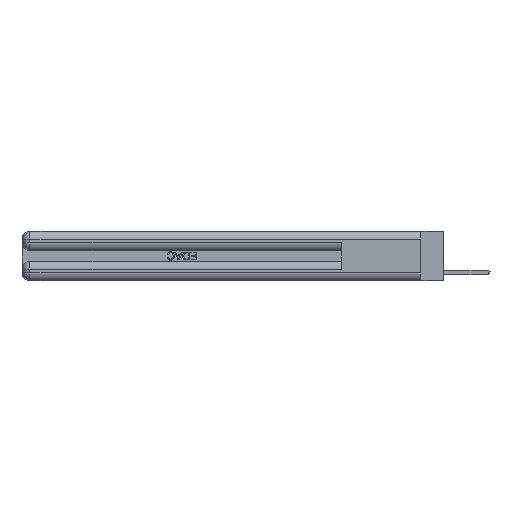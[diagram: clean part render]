
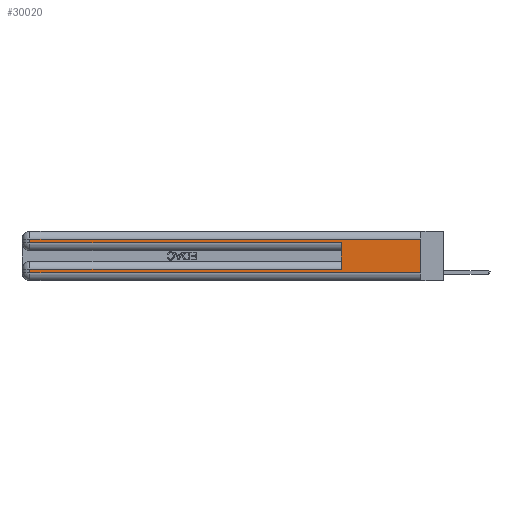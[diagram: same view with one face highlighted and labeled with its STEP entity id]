
A CAD part, left-side view. The second image highlights one B-rep face of the part: STEP entity #30020.
In plain terms, the highlighted planar face has unit normal (-1, 0, 0).
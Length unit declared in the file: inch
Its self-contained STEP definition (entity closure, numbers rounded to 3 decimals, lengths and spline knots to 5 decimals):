
#575 = ORIENTED_EDGE ( 'NONE', *, *, #23349, .F. ) ;
#660 = DIRECTION ( 'NONE',  ( 0., 0., 1. ) ) ;
#1958 = ORIENTED_EDGE ( 'NONE', *, *, #13473, .T. ) ;
#2178 = EDGE_CURVE ( 'NONE', #5059, #28008, #10118, .T. ) ;
#2394 = VECTOR ( 'NONE', #660, 39.37008 ) ;
#2495 = LINE ( 'NONE', #28768, #8715 ) ;
#2496 = FACE_OUTER_BOUND ( 'NONE', #28478, .T. ) ;
#2797 = CARTESIAN_POINT ( 'NONE',  ( 0., 0.6, 0.145 ) ) ;
#2930 = DIRECTION ( 'NONE',  ( 0., -1., 0. ) ) ;
#3927 = DIRECTION ( 'NONE',  ( 0., 0., -1. ) ) ;
#5059 = VERTEX_POINT ( 'NONE', #8813 ) ;
#5976 = CARTESIAN_POINT ( 'NONE',  ( 0., 2.94, 0.37 ) ) ;
#6125 = DIRECTION ( 'NONE',  ( 0., 0., -1. ) ) ;
#7671 = EDGE_CURVE ( 'NONE', #9877, #20302, #30040, .T. ) ;
#7753 = CARTESIAN_POINT ( 'NONE',  ( 0., 2.94, 0.285 ) ) ;
#7903 = CARTESIAN_POINT ( 'NONE',  ( 0., 0., 0.085 ) ) ;
#8715 = VECTOR ( 'NONE', #10646, 39.37008 ) ;
#8813 = CARTESIAN_POINT ( 'NONE',  ( 0., 0.6, 0.085 ) ) ;
#9092 = DIRECTION ( 'NONE',  ( 0., -1., 0. ) ) ;
#9561 = DIRECTION ( 'NONE',  ( 0., 1., 0. ) ) ;
#9877 = VERTEX_POINT ( 'NONE', #28193 ) ;
#10118 = LINE ( 'NONE', #7903, #12491 ) ;
#10181 = DIRECTION ( 'NONE',  ( 1., 0., 0. ) ) ;
#10646 = DIRECTION ( 'NONE',  ( 0., 0., -1. ) ) ;
#11634 = ORIENTED_EDGE ( 'NONE', *, *, #19219, .T. ) ;
#12491 = VECTOR ( 'NONE', #15438, 39.37008 ) ;
#12512 = CARTESIAN_POINT ( 'NONE',  ( 0., 0., 0.37 ) ) ;
#12623 = ORIENTED_EDGE ( 'NONE', *, *, #7671, .F. ) ;
#13065 = ORIENTED_EDGE ( 'NONE', *, *, #20601, .T. ) ;
#13370 = VECTOR ( 'NONE', #9092, 39.37008 ) ;
#13473 = EDGE_CURVE ( 'NONE', #28131, #22437, #15703, .T. ) ;
#15438 = DIRECTION ( 'NONE',  ( 0., 1., 0. ) ) ;
#15703 = LINE ( 'NONE', #5976, #20096 ) ;
#16310 = VECTOR ( 'NONE', #9561, 39.37008 ) ;
#16314 = CARTESIAN_POINT ( 'NONE',  ( 0., 0., 0.285 ) ) ;
#17798 = VERTEX_POINT ( 'NONE', #25293 ) ;
#18043 = EDGE_CURVE ( 'NONE', #17798, #20302, #19240, .T. ) ;
#18176 = EDGE_CURVE ( 'NONE', #28008, #17798, #2495, .T. ) ;
#18614 = AXIS2_PLACEMENT_3D ( 'NONE', #12512, #10181, #26714 ) ;
#19219 = EDGE_CURVE ( 'NONE', #9877, #28131, #23289, .T. ) ;
#19240 = LINE ( 'NONE', #26866, #30184 ) ;
#19350 = ORIENTED_EDGE ( 'NONE', *, *, #2178, .T. ) ;
#20096 = VECTOR ( 'NONE', #6125, 39.37008 ) ;
#20302 = VERTEX_POINT ( 'NONE', #21498 ) ;
#20580 = ORIENTED_EDGE ( 'NONE', *, *, #18176, .T. ) ;
#20601 = EDGE_CURVE ( 'NONE', #22437, #27794, #21268, .T. ) ;
#20970 = CARTESIAN_POINT ( 'NONE',  ( 0., 0., 0.37 ) ) ;
#21268 = LINE ( 'NONE', #16314, #13370 ) ;
#21498 = CARTESIAN_POINT ( 'NONE',  ( 0., 0., 0.06 ) ) ;
#22437 = VERTEX_POINT ( 'NONE', #7753 ) ;
#23289 = LINE ( 'NONE', #23753, #16310 ) ;
#23349 = EDGE_CURVE ( 'NONE', #5059, #27794, #24363, .T. ) ;
#23753 = CARTESIAN_POINT ( 'NONE',  ( 0., 0., 0.31 ) ) ;
#23778 = CARTESIAN_POINT ( 'NONE',  ( 0., 2.94, 0.31 ) ) ;
#23960 = CARTESIAN_POINT ( 'NONE',  ( 0., 0.6, 0.285 ) ) ;
#24363 = LINE ( 'NONE', #2797, #2394 ) ;
#25293 = CARTESIAN_POINT ( 'NONE',  ( 0., 2.94, 0.06 ) ) ;
#26714 = DIRECTION ( 'NONE',  ( 0., 0., -1. ) ) ;
#26866 = CARTESIAN_POINT ( 'NONE',  ( 0., 0., 0.06 ) ) ;
#27392 = CARTESIAN_POINT ( 'NONE',  ( 0., 2.94, 0.085 ) ) ;
#27794 = VERTEX_POINT ( 'NONE', #23960 ) ;
#28008 = VERTEX_POINT ( 'NONE', #27392 ) ;
#28131 = VERTEX_POINT ( 'NONE', #23778 ) ;
#28193 = CARTESIAN_POINT ( 'NONE',  ( 0., 0., 0.31 ) ) ;
#28478 = EDGE_LOOP ( 'NONE', ( #12623, #11634, #1958, #13065, #575, #19350, #20580, #29273 ) ) ;
#28768 = CARTESIAN_POINT ( 'NONE',  ( 0., 2.94, 0.37 ) ) ;
#28875 = VECTOR ( 'NONE', #3927, 39.37008 ) ;
#28909 = PLANE ( 'NONE',  #18614 ) ;
#29273 = ORIENTED_EDGE ( 'NONE', *, *, #18043, .T. ) ;
#30020 = ADVANCED_FACE ( 'NONE', ( #2496 ), #28909, .F. ) ;
#30040 = LINE ( 'NONE', #20970, #28875 ) ;
#30184 = VECTOR ( 'NONE', #2930, 39.37008 ) ;
